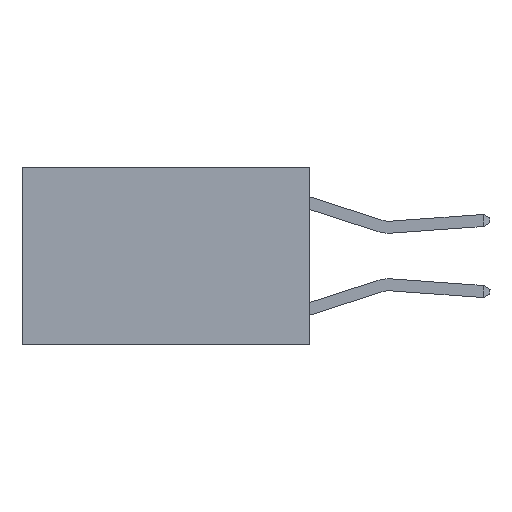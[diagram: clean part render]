
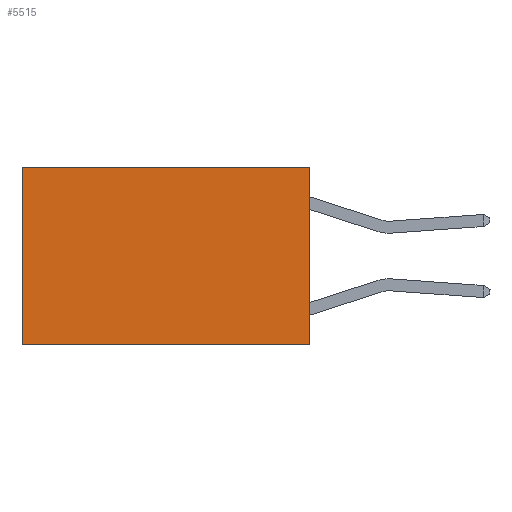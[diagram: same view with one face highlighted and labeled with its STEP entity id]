
A CAD part, left-side view. The second image highlights one B-rep face of the part: STEP entity #5515.
In plain terms, the highlighted planar face has unit normal (-1, 0, 0).
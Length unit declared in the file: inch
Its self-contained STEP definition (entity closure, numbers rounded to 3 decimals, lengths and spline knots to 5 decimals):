
#194 = DIRECTION ( 'NONE',  ( 1., 0., 0. ) ) ;
#3118 = VECTOR ( 'NONE', #13965, 39.37008 ) ;
#3247 = ORIENTED_EDGE ( 'NONE', *, *, #21756, .F. ) ;
#3899 = LINE ( 'NONE', #6781, #3118 ) ;
#4370 = ORIENTED_EDGE ( 'NONE', *, *, #19569, .F. ) ;
#5515 = ADVANCED_FACE ( 'NONE', ( #14279 ), #28735, .F. ) ;
#6045 = DIRECTION ( 'NONE',  ( 0., 1., 0. ) ) ;
#6243 = VECTOR ( 'NONE', #15960, 39.37008 ) ;
#6781 = CARTESIAN_POINT ( 'NONE',  ( 0.2625, 0., 0. ) ) ;
#7395 = CARTESIAN_POINT ( 'NONE',  ( 0.2625, 0., 0. ) ) ;
#10287 = LINE ( 'NONE', #25042, #28585 ) ;
#10541 = CARTESIAN_POINT ( 'NONE',  ( 0.2625, 0.6, -0.37 ) ) ;
#11554 = VERTEX_POINT ( 'NONE', #30635 ) ;
#12941 = EDGE_LOOP ( 'NONE', ( #24428, #4370, #3247, #16651 ) ) ;
#13029 = DIRECTION ( 'NONE',  ( 0., 1., 0. ) ) ;
#13678 = VERTEX_POINT ( 'NONE', #17314 ) ;
#13965 = DIRECTION ( 'NONE',  ( 0., 0., -1. ) ) ;
#14279 = FACE_OUTER_BOUND ( 'NONE', #12941, .T. ) ;
#15960 = DIRECTION ( 'NONE',  ( 0., 0., -1. ) ) ;
#16651 = ORIENTED_EDGE ( 'NONE', *, *, #17137, .T. ) ;
#16947 = DIRECTION ( 'NONE',  ( 0., 0., -1. ) ) ;
#17137 = EDGE_CURVE ( 'NONE', #13678, #23981, #27650, .T. ) ;
#17314 = CARTESIAN_POINT ( 'NONE',  ( 0.2625, 0., 0. ) ) ;
#17824 = CARTESIAN_POINT ( 'NONE',  ( 0.2625, 0., 0. ) ) ;
#18257 = CARTESIAN_POINT ( 'NONE',  ( 0.2625, 0.6, 0. ) ) ;
#18387 = VERTEX_POINT ( 'NONE', #10541 ) ;
#19569 = EDGE_CURVE ( 'NONE', #11554, #18387, #10287, .T. ) ;
#19734 = AXIS2_PLACEMENT_3D ( 'NONE', #7395, #194, #16947 ) ;
#21756 = EDGE_CURVE ( 'NONE', #13678, #11554, #3899, .T. ) ;
#22185 = CARTESIAN_POINT ( 'NONE',  ( 0.2625, 0.6, 0. ) ) ;
#23553 = EDGE_CURVE ( 'NONE', #23981, #18387, #25300, .T. ) ;
#23981 = VERTEX_POINT ( 'NONE', #22185 ) ;
#24428 = ORIENTED_EDGE ( 'NONE', *, *, #23553, .T. ) ;
#25042 = CARTESIAN_POINT ( 'NONE',  ( 0.2625, 0., -0.37 ) ) ;
#25300 = LINE ( 'NONE', #18257, #6243 ) ;
#26886 = VECTOR ( 'NONE', #13029, 39.37008 ) ;
#27650 = LINE ( 'NONE', #17824, #26886 ) ;
#28585 = VECTOR ( 'NONE', #6045, 39.37008 ) ;
#28735 = PLANE ( 'NONE',  #19734 ) ;
#30635 = CARTESIAN_POINT ( 'NONE',  ( 0.2625, 0., -0.37 ) ) ;
